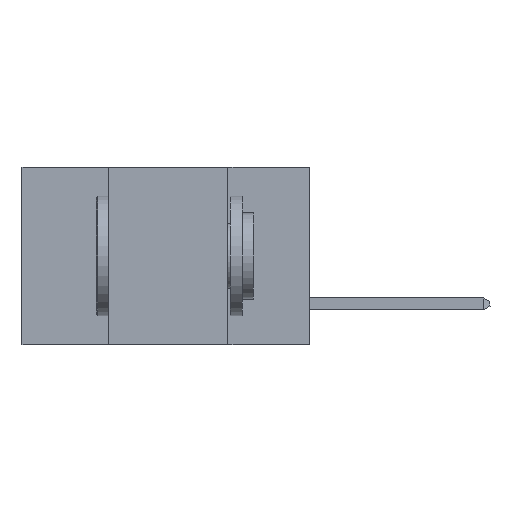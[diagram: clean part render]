
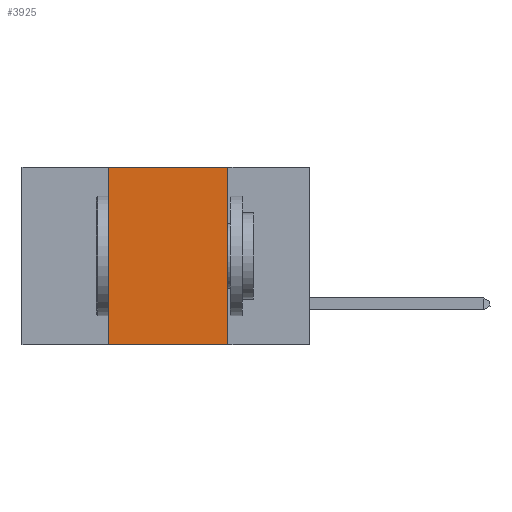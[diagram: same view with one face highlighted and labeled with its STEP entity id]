
A CAD part, left-side view. The second image highlights one B-rep face of the part: STEP entity #3925.
In plain terms, the highlighted planar face has unit normal (-1, 0, 0).
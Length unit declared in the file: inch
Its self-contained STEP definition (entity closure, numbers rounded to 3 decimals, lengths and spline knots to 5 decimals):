
#860 = VERTEX_POINT ( 'NONE', #9689 ) ;
#1998 = DIRECTION ( 'NONE',  ( 0., 0., -1. ) ) ;
#2921 = AXIS2_PLACEMENT_3D ( 'NONE', #10436, #10404, #6022 ) ;
#3241 = EDGE_CURVE ( 'NONE', #860, #9178, #10558, .T. ) ;
#3498 = DIRECTION ( 'NONE',  ( 0., -1., 0. ) ) ;
#3562 = VERTEX_POINT ( 'NONE', #11350 ) ;
#3632 = FACE_OUTER_BOUND ( 'NONE', #8082, .T. ) ;
#3854 = VECTOR ( 'NONE', #3498, 39.37008 ) ;
#3925 = ADVANCED_FACE ( 'NONE', ( #3632 ), #9637, .F. ) ;
#4196 = EDGE_CURVE ( 'NONE', #3562, #6042, #9280, .T. ) ;
#4208 = CARTESIAN_POINT ( 'NONE',  ( 0., 0.17, -0.37 ) ) ;
#4272 = CARTESIAN_POINT ( 'NONE',  ( 0., 0.42, 0. ) ) ;
#4901 = ORIENTED_EDGE ( 'NONE', *, *, #10074, .F. ) ;
#5833 = DIRECTION ( 'NONE',  ( 0., 0., 1. ) ) ;
#6022 = DIRECTION ( 'NONE',  ( 0., 0., -1. ) ) ;
#6042 = VERTEX_POINT ( 'NONE', #4208 ) ;
#6059 = ORIENTED_EDGE ( 'NONE', *, *, #3241, .F. ) ;
#6196 = CARTESIAN_POINT ( 'NONE',  ( 0., 0.6, 0. ) ) ;
#6536 = DIRECTION ( 'NONE',  ( 0., -1., 0. ) ) ;
#6625 = LINE ( 'NONE', #6196, #3854 ) ;
#7391 = EDGE_CURVE ( 'NONE', #860, #6042, #9524, .T. ) ;
#8082 = EDGE_LOOP ( 'NONE', ( #11255, #4901, #6059, #10609 ) ) ;
#8198 = CARTESIAN_POINT ( 'NONE',  ( 0., 0.6, -0.37 ) ) ;
#8224 = CARTESIAN_POINT ( 'NONE',  ( 0., 0.42, 0. ) ) ;
#9034 = CARTESIAN_POINT ( 'NONE',  ( 0., 0.17, 0. ) ) ;
#9178 = VERTEX_POINT ( 'NONE', #4272 ) ;
#9280 = LINE ( 'NONE', #9034, #9841 ) ;
#9524 = LINE ( 'NONE', #8198, #10472 ) ;
#9637 = PLANE ( 'NONE',  #2921 ) ;
#9689 = CARTESIAN_POINT ( 'NONE',  ( 0., 0.42, -0.37 ) ) ;
#9737 = VECTOR ( 'NONE', #5833, 39.37008 ) ;
#9841 = VECTOR ( 'NONE', #1998, 39.37008 ) ;
#10074 = EDGE_CURVE ( 'NONE', #9178, #3562, #6625, .T. ) ;
#10404 = DIRECTION ( 'NONE',  ( 1., 0., 0. ) ) ;
#10436 = CARTESIAN_POINT ( 'NONE',  ( 0., 0.6, 0. ) ) ;
#10472 = VECTOR ( 'NONE', #6536, 39.37008 ) ;
#10558 = LINE ( 'NONE', #8224, #9737 ) ;
#10609 = ORIENTED_EDGE ( 'NONE', *, *, #7391, .T. ) ;
#11255 = ORIENTED_EDGE ( 'NONE', *, *, #4196, .F. ) ;
#11350 = CARTESIAN_POINT ( 'NONE',  ( 0., 0.17, 0. ) ) ;
